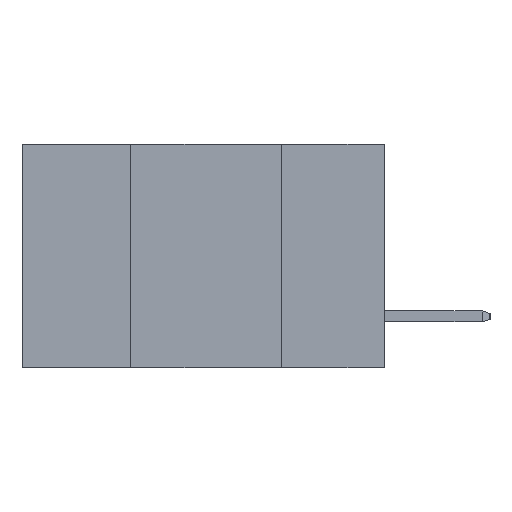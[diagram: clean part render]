
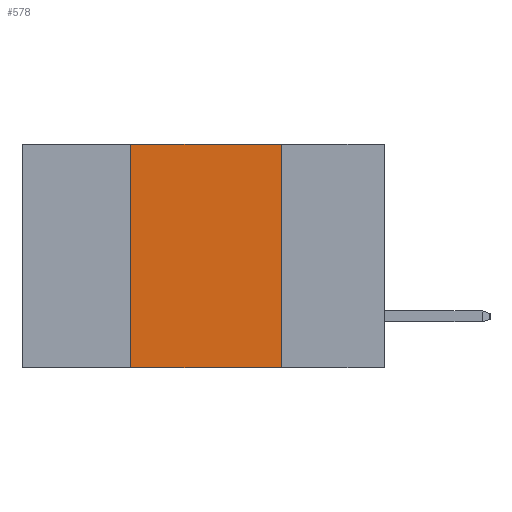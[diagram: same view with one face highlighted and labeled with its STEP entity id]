
A CAD part, left-side view. The second image highlights one B-rep face of the part: STEP entity #578.
In plain terms, the highlighted planar face has unit normal (-1, 0, 0).
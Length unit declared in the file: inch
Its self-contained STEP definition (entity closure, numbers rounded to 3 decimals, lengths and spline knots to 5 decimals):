
#251 = LINE ( 'NONE', #6771, #8979 ) ;
#578 = ADVANCED_FACE ( 'NONE', ( #8100 ), #8021, .F. ) ;
#1173 = AXIS2_PLACEMENT_3D ( 'NONE', #7847, #8749, #8702 ) ;
#1262 = VECTOR ( 'NONE', #9169, 39.37008 ) ;
#1286 = EDGE_CURVE ( 'NONE', #6562, #10519, #4317, .T. ) ;
#2833 = VERTEX_POINT ( 'NONE', #8087 ) ;
#2904 = ORIENTED_EDGE ( 'NONE', *, *, #8537, .F. ) ;
#3047 = CARTESIAN_POINT ( 'NONE',  ( 0., 0.17, 0. ) ) ;
#3104 = EDGE_CURVE ( 'NONE', #5533, #2833, #251, .T. ) ;
#4055 = VECTOR ( 'NONE', #7330, 39.37008 ) ;
#4273 = LINE ( 'NONE', #8378, #1262 ) ;
#4317 = LINE ( 'NONE', #8070, #4055 ) ;
#4474 = CARTESIAN_POINT ( 'NONE',  ( 0., 0.42, 0. ) ) ;
#4659 = ORIENTED_EDGE ( 'NONE', *, *, #1286, .F. ) ;
#4822 = CARTESIAN_POINT ( 'NONE',  ( 0., 0.42, -0.37 ) ) ;
#4830 = DIRECTION ( 'NONE',  ( 0., 0., 1. ) ) ;
#5533 = VERTEX_POINT ( 'NONE', #10032 ) ;
#6107 = LINE ( 'NONE', #4822, #10085 ) ;
#6562 = VERTEX_POINT ( 'NONE', #4474 ) ;
#6628 = EDGE_CURVE ( 'NONE', #5533, #6562, #6107, .T. ) ;
#6771 = CARTESIAN_POINT ( 'NONE',  ( 0., 0.6, -0.37 ) ) ;
#7330 = DIRECTION ( 'NONE',  ( 0., -1., 0. ) ) ;
#7847 = CARTESIAN_POINT ( 'NONE',  ( 0., 0.6, 0. ) ) ;
#8021 = PLANE ( 'NONE',  #1173 ) ;
#8070 = CARTESIAN_POINT ( 'NONE',  ( 0., 0.6, 0. ) ) ;
#8087 = CARTESIAN_POINT ( 'NONE',  ( 0., 0.17, -0.37 ) ) ;
#8100 = FACE_OUTER_BOUND ( 'NONE', #10832, .T. ) ;
#8283 = ORIENTED_EDGE ( 'NONE', *, *, #3104, .T. ) ;
#8378 = CARTESIAN_POINT ( 'NONE',  ( 0., 0.17, -0.37 ) ) ;
#8520 = ORIENTED_EDGE ( 'NONE', *, *, #6628, .F. ) ;
#8537 = EDGE_CURVE ( 'NONE', #10519, #2833, #4273, .T. ) ;
#8702 = DIRECTION ( 'NONE',  ( 0., 0., -1. ) ) ;
#8749 = DIRECTION ( 'NONE',  ( 1., 0., 0. ) ) ;
#8979 = VECTOR ( 'NONE', #9163, 39.37008 ) ;
#9163 = DIRECTION ( 'NONE',  ( 0., -1., 0. ) ) ;
#9169 = DIRECTION ( 'NONE',  ( 0., 0., -1. ) ) ;
#10032 = CARTESIAN_POINT ( 'NONE',  ( 0., 0.42, -0.37 ) ) ;
#10085 = VECTOR ( 'NONE', #4830, 39.37008 ) ;
#10519 = VERTEX_POINT ( 'NONE', #3047 ) ;
#10832 = EDGE_LOOP ( 'NONE', ( #2904, #4659, #8520, #8283 ) ) ;
